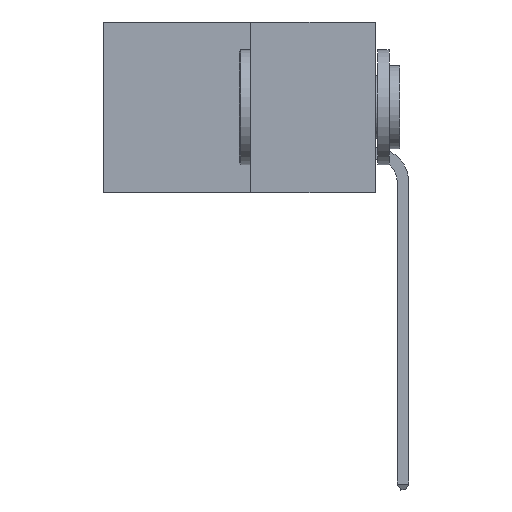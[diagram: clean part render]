
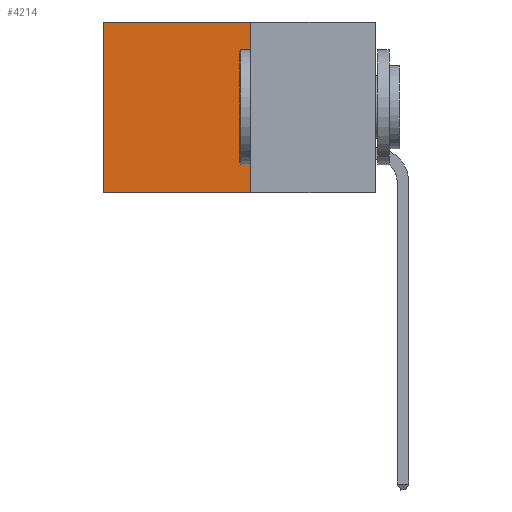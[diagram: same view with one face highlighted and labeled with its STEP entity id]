
A CAD part, left-side view. The second image highlights one B-rep face of the part: STEP entity #4214.
In plain terms, the highlighted planar face has unit normal (-1, 0, 0).
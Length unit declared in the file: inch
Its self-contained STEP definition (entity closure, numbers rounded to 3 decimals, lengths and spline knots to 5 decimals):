
#19 = DIRECTION ( 'NONE',  ( 0., 0., -1. ) ) ;
#610 = ORIENTED_EDGE ( 'NONE', *, *, #832, .F. ) ;
#832 = EDGE_CURVE ( 'NONE', #1685, #7342, #8255, .T. ) ;
#1685 = VERTEX_POINT ( 'NONE', #5468 ) ;
#1736 = VECTOR ( 'NONE', #19, 39.37008 ) ;
#1775 = LINE ( 'NONE', #4540, #3644 ) ;
#1972 = LINE ( 'NONE', #6977, #7883 ) ;
#2133 = CARTESIAN_POINT ( 'NONE',  ( 0.277, 0.59, -0.37 ) ) ;
#2591 = CARTESIAN_POINT ( 'NONE',  ( 0.277, 0.27, -0.37 ) ) ;
#2947 = ORIENTED_EDGE ( 'NONE', *, *, #8645, .T. ) ;
#3030 = CARTESIAN_POINT ( 'NONE',  ( 0.277, 0.27, -0.37 ) ) ;
#3644 = VECTOR ( 'NONE', #4524, 39.37008 ) ;
#3992 = VECTOR ( 'NONE', #7188, 39.37008 ) ;
#4010 = VERTEX_POINT ( 'NONE', #5373 ) ;
#4099 = EDGE_CURVE ( 'NONE', #7342, #7974, #1972, .T. ) ;
#4113 = CARTESIAN_POINT ( 'NONE',  ( 0.277, 0.27, -0.37 ) ) ;
#4214 = ADVANCED_FACE ( 'NONE', ( #8411 ), #4396, .F. ) ;
#4339 = DIRECTION ( 'NONE',  ( 1., 0., 0. ) ) ;
#4396 = PLANE ( 'NONE',  #7424 ) ;
#4524 = DIRECTION ( 'NONE',  ( 0., 1., 0. ) ) ;
#4540 = CARTESIAN_POINT ( 'NONE',  ( 0.277, 0.27, 0. ) ) ;
#4847 = DIRECTION ( 'NONE',  ( 0., 0., -1. ) ) ;
#5373 = CARTESIAN_POINT ( 'NONE',  ( 0.277, 0.59, 0. ) ) ;
#5468 = CARTESIAN_POINT ( 'NONE',  ( 0.277, 0.27, 0. ) ) ;
#6241 = CARTESIAN_POINT ( 'NONE',  ( 0.277, 0.59, -0.37 ) ) ;
#6337 = ORIENTED_EDGE ( 'NONE', *, *, #7011, .T. ) ;
#6796 = DIRECTION ( 'NONE',  ( 0., 1., 0. ) ) ;
#6977 = CARTESIAN_POINT ( 'NONE',  ( 0.277, 0.27, -0.37 ) ) ;
#7011 = EDGE_CURVE ( 'NONE', #1685, #4010, #1775, .T. ) ;
#7188 = DIRECTION ( 'NONE',  ( 0., 0., -1. ) ) ;
#7342 = VERTEX_POINT ( 'NONE', #2591 ) ;
#7424 = AXIS2_PLACEMENT_3D ( 'NONE', #4113, #4339, #4847 ) ;
#7883 = VECTOR ( 'NONE', #6796, 39.37008 ) ;
#7974 = VERTEX_POINT ( 'NONE', #2133 ) ;
#8095 = EDGE_LOOP ( 'NONE', ( #2947, #9065, #610, #6337 ) ) ;
#8255 = LINE ( 'NONE', #3030, #3992 ) ;
#8411 = FACE_OUTER_BOUND ( 'NONE', #8095, .T. ) ;
#8645 = EDGE_CURVE ( 'NONE', #4010, #7974, #9449, .T. ) ;
#9065 = ORIENTED_EDGE ( 'NONE', *, *, #4099, .F. ) ;
#9449 = LINE ( 'NONE', #6241, #1736 ) ;
